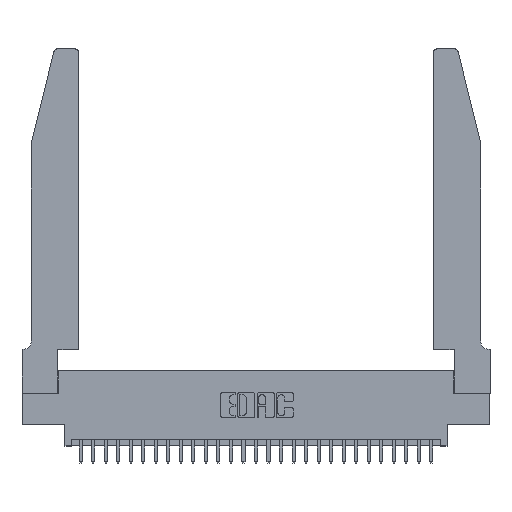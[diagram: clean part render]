
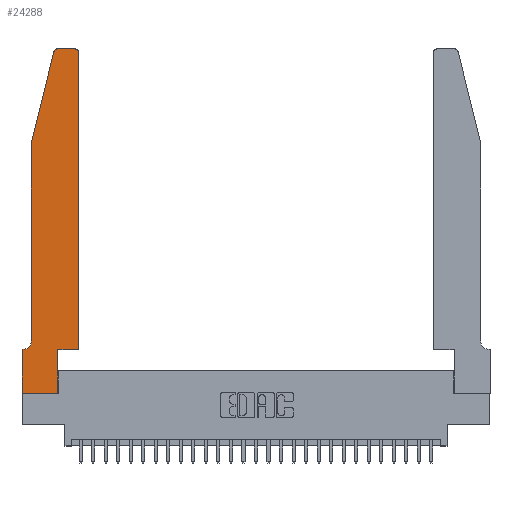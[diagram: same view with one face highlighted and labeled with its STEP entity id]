
A CAD part, top view. The second image highlights one B-rep face of the part: STEP entity #24288.
In plain terms, the highlighted planar face has unit normal (0, 0, 1).
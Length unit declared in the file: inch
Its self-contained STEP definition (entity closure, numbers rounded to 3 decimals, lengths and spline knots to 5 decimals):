
#149 = AXIS2_PLACEMENT_3D ( 'NONE', #4648, #8843, #17976 ) ;
#173 = EDGE_CURVE ( 'NONE', #22189, #19795, #18890, .T. ) ;
#560 = DIRECTION ( 'NONE',  ( 0., 0., 1. ) ) ;
#685 = ORIENTED_EDGE ( 'NONE', *, *, #16003, .T. ) ;
#724 = CARTESIAN_POINT ( 'NONE',  ( 0., 0., 0.37 ) ) ;
#983 = CARTESIAN_POINT ( 'NONE',  ( 0.4505, 2.72, 0.37 ) ) ;
#1225 = CARTESIAN_POINT ( 'NONE',  ( 0., 0., 0.37 ) ) ;
#1650 = DIRECTION ( 'NONE',  ( 0., -1., 0. ) ) ;
#1692 = ORIENTED_EDGE ( 'NONE', *, *, #17974, .T. ) ;
#1826 = LINE ( 'NONE', #21493, #19869 ) ;
#2147 = ORIENTED_EDGE ( 'NONE', *, *, #9199, .T. ) ;
#2648 = DIRECTION ( 'NONE',  ( 0., 1., 0. ) ) ;
#2828 = ORIENTED_EDGE ( 'NONE', *, *, #6555, .T. ) ;
#2934 = CARTESIAN_POINT ( 'NONE',  ( 0.2865, 0.35, 0.37 ) ) ;
#3142 = VECTOR ( 'NONE', #2648, 39.37008 ) ;
#3515 = VECTOR ( 'NONE', #1650, 39.37008 ) ;
#4648 = CARTESIAN_POINT ( 'NONE',  ( 0., 0.35, 0.37 ) ) ;
#4700 = VERTEX_POINT ( 'NONE', #1225 ) ;
#4862 = EDGE_CURVE ( 'NONE', #24119, #7692, #13163, .T. ) ;
#5092 = EDGE_LOOP ( 'NONE', ( #12367, #28994, #18056, #2147, #22766, #21688, #685, #2828, #1692, #21113, #15904, #10833 ) ) ;
#5913 = LINE ( 'NONE', #2934, #22560 ) ;
#6460 = LINE ( 'NONE', #7829, #21334 ) ;
#6546 = EDGE_CURVE ( 'NONE', #17114, #15315, #15559, .T. ) ;
#6555 = EDGE_CURVE ( 'NONE', #4700, #9228, #25896, .T. ) ;
#6683 = EDGE_CURVE ( 'NONE', #24160, #17114, #21927, .T. ) ;
#6691 = CARTESIAN_POINT ( 'NONE',  ( 0.284, 2.72, 0.37 ) ) ;
#7369 = DIRECTION ( 'NONE',  ( 1., 0., 0. ) ) ;
#7692 = VERTEX_POINT ( 'NONE', #13351 ) ;
#7829 = CARTESIAN_POINT ( 'NONE',  ( 0.0755, 2., 0.37 ) ) ;
#8823 = CARTESIAN_POINT ( 'NONE',  ( 0.4205, 2.75, 0.37 ) ) ;
#8843 = DIRECTION ( 'NONE',  ( 0., 0., 1. ) ) ;
#9199 = EDGE_CURVE ( 'NONE', #27521, #16575, #20709, .T. ) ;
#9228 = VERTEX_POINT ( 'NONE', #14310 ) ;
#9367 = EDGE_CURVE ( 'NONE', #15315, #22189, #27522, .T. ) ;
#9552 = LINE ( 'NONE', #29067, #3515 ) ;
#10236 = AXIS2_PLACEMENT_3D ( 'NONE', #6691, #20434, #7369 ) ;
#10354 = CARTESIAN_POINT ( 'NONE',  ( 0.2865, 0.35, 0.37 ) ) ;
#10833 = ORIENTED_EDGE ( 'NONE', *, *, #6546, .T. ) ;
#11182 = PLANE ( 'NONE',  #149 ) ;
#12367 = ORIENTED_EDGE ( 'NONE', *, *, #9367, .T. ) ;
#12727 = CARTESIAN_POINT ( 'NONE',  ( 0.0755, 0.42, 0.37 ) ) ;
#13163 = LINE ( 'NONE', #14151, #21665 ) ;
#13351 = CARTESIAN_POINT ( 'NONE',  ( 0., 0.35, 0.37 ) ) ;
#14151 = CARTESIAN_POINT ( 'NONE',  ( 0.0755, 0.35, 0.37 ) ) ;
#14310 = CARTESIAN_POINT ( 'NONE',  ( 0.2865, 0., 0.37 ) ) ;
#14659 = DIRECTION ( 'NONE',  ( -0.239, -0.971, 0. ) ) ;
#14690 = VECTOR ( 'NONE', #26827, 39.37008 ) ;
#14763 = CIRCLE ( 'NONE', #28396, 0.07 ) ;
#15099 = EDGE_CURVE ( 'NONE', #16633, #24160, #1826, .T. ) ;
#15315 = VERTEX_POINT ( 'NONE', #8823 ) ;
#15559 = CIRCLE ( 'NONE', #19577, 0.03 ) ;
#15904 = ORIENTED_EDGE ( 'NONE', *, *, #6683, .T. ) ;
#15916 = CARTESIAN_POINT ( 'NONE',  ( 0.0055, 0.42, 0.37 ) ) ;
#16003 = EDGE_CURVE ( 'NONE', #7692, #4700, #9552, .T. ) ;
#16403 = CARTESIAN_POINT ( 'NONE',  ( 0.4505, 0.35, 0.37 ) ) ;
#16575 = VERTEX_POINT ( 'NONE', #12727 ) ;
#16633 = VERTEX_POINT ( 'NONE', #10354 ) ;
#17114 = VERTEX_POINT ( 'NONE', #983 ) ;
#17132 = DIRECTION ( 'NONE',  ( 1., 0., 0. ) ) ;
#17233 = FACE_OUTER_BOUND ( 'NONE', #5092, .T. ) ;
#17508 = VECTOR ( 'NONE', #19214, 39.37008 ) ;
#17759 = EDGE_CURVE ( 'NONE', #16575, #24119, #14763, .T. ) ;
#17974 = EDGE_CURVE ( 'NONE', #9228, #16633, #5913, .T. ) ;
#17976 = DIRECTION ( 'NONE',  ( 1., 0., 0. ) ) ;
#18056 = ORIENTED_EDGE ( 'NONE', *, *, #20996, .T. ) ;
#18191 = DIRECTION ( 'NONE',  ( 1., 0., 0. ) ) ;
#18544 = DIRECTION ( 'NONE',  ( 1., 0., 0. ) ) ;
#18890 = CIRCLE ( 'NONE', #10236, 0.03 ) ;
#18932 = CARTESIAN_POINT ( 'NONE',  ( 0.0755, 2., 0.37 ) ) ;
#19214 = DIRECTION ( 'NONE',  ( 0., -1., 0. ) ) ;
#19577 = AXIS2_PLACEMENT_3D ( 'NONE', #25366, #560, #18191 ) ;
#19715 = CARTESIAN_POINT ( 'NONE',  ( 0.2605, 2.75, 0.37 ) ) ;
#19795 = VERTEX_POINT ( 'NONE', #28147 ) ;
#19869 = VECTOR ( 'NONE', #17132, 39.37008 ) ;
#20024 = CARTESIAN_POINT ( 'NONE',  ( 0.0755, 2., 0.37 ) ) ;
#20049 = DIRECTION ( 'NONE',  ( 0., 0., -1. ) ) ;
#20391 = CARTESIAN_POINT ( 'NONE',  ( 0.284, 2.75, 0.37 ) ) ;
#20434 = DIRECTION ( 'NONE',  ( 0., 0., 1. ) ) ;
#20709 = LINE ( 'NONE', #18932, #17508 ) ;
#20996 = EDGE_CURVE ( 'NONE', #19795, #27521, #6460, .T. ) ;
#21113 = ORIENTED_EDGE ( 'NONE', *, *, #15099, .T. ) ;
#21334 = VECTOR ( 'NONE', #14659, 39.37008 ) ;
#21493 = CARTESIAN_POINT ( 'NONE',  ( 0.4505, 0.35, 0.37 ) ) ;
#21665 = VECTOR ( 'NONE', #25570, 39.37008 ) ;
#21688 = ORIENTED_EDGE ( 'NONE', *, *, #4862, .T. ) ;
#21927 = LINE ( 'NONE', #16403, #3142 ) ;
#22189 = VERTEX_POINT ( 'NONE', #20391 ) ;
#22560 = VECTOR ( 'NONE', #28240, 39.37008 ) ;
#22766 = ORIENTED_EDGE ( 'NONE', *, *, #17759, .T. ) ;
#24119 = VERTEX_POINT ( 'NONE', #25902 ) ;
#24160 = VERTEX_POINT ( 'NONE', #26781 ) ;
#24288 = ADVANCED_FACE ( 'NONE', ( #17233 ), #11182, .T. ) ;
#25183 = VECTOR ( 'NONE', #18544, 39.37008 ) ;
#25366 = CARTESIAN_POINT ( 'NONE',  ( 0.4205, 2.72, 0.37 ) ) ;
#25570 = DIRECTION ( 'NONE',  ( -1., 0., 0. ) ) ;
#25896 = LINE ( 'NONE', #724, #25183 ) ;
#25902 = CARTESIAN_POINT ( 'NONE',  ( 0.0055, 0.35, 0.37 ) ) ;
#26781 = CARTESIAN_POINT ( 'NONE',  ( 0.4505, 0.35, 0.37 ) ) ;
#26827 = DIRECTION ( 'NONE',  ( -1., 0., 0. ) ) ;
#26979 = DIRECTION ( 'NONE',  ( -1., 0., 0. ) ) ;
#27521 = VERTEX_POINT ( 'NONE', #20024 ) ;
#27522 = LINE ( 'NONE', #19715, #14690 ) ;
#28147 = CARTESIAN_POINT ( 'NONE',  ( 0.25487, 2.72718, 0.37 ) ) ;
#28240 = DIRECTION ( 'NONE',  ( 0., 1., 0. ) ) ;
#28396 = AXIS2_PLACEMENT_3D ( 'NONE', #15916, #20049, #26979 ) ;
#28994 = ORIENTED_EDGE ( 'NONE', *, *, #173, .T. ) ;
#29067 = CARTESIAN_POINT ( 'NONE',  ( 0., 0., 0.37 ) ) ;
